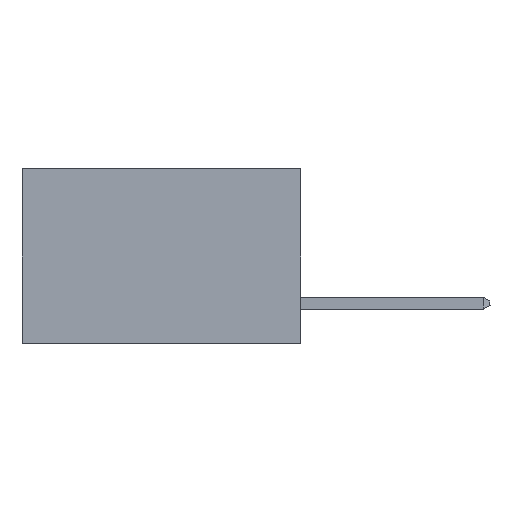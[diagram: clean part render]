
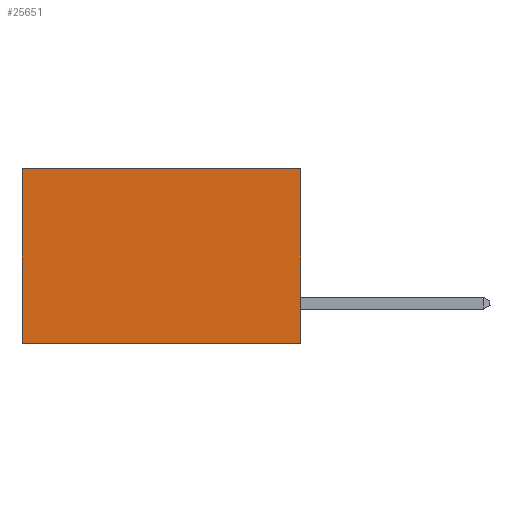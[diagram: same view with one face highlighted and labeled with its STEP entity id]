
A CAD part, left-side view. The second image highlights one B-rep face of the part: STEP entity #25651.
In plain terms, the highlighted planar face has unit normal (-1, 0, 0).
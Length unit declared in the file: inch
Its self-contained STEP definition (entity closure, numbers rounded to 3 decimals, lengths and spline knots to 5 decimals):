
#2387 = DIRECTION ( 'NONE',  ( 0., 0., -1. ) ) ;
#3054 = LINE ( 'NONE', #18910, #8202 ) ;
#3351 = EDGE_CURVE ( 'NONE', #3638, #4696, #25672, .T. ) ;
#3638 = VERTEX_POINT ( 'NONE', #5521 ) ;
#4696 = VERTEX_POINT ( 'NONE', #24232 ) ;
#5521 = CARTESIAN_POINT ( 'NONE',  ( 0.277, 0.59, 0. ) ) ;
#5921 = EDGE_CURVE ( 'NONE', #14532, #13991, #19021, .T. ) ;
#8202 = VECTOR ( 'NONE', #10295, 39.37008 ) ;
#9081 = DIRECTION ( 'NONE',  ( 0., 1., 0. ) ) ;
#9357 = CARTESIAN_POINT ( 'NONE',  ( 0.277, 0., -0.37 ) ) ;
#9392 = DIRECTION ( 'NONE',  ( 0., 0., -1. ) ) ;
#10214 = CARTESIAN_POINT ( 'NONE',  ( 0.277, 0., -0.37 ) ) ;
#10295 = DIRECTION ( 'NONE',  ( 0., 1., 0. ) ) ;
#11692 = ORIENTED_EDGE ( 'NONE', *, *, #3351, .T. ) ;
#12335 = DIRECTION ( 'NONE',  ( 0., 0., -1. ) ) ;
#12855 = EDGE_CURVE ( 'NONE', #13991, #4696, #24137, .T. ) ;
#13382 = VECTOR ( 'NONE', #2387, 39.37008 ) ;
#13991 = VERTEX_POINT ( 'NONE', #21744 ) ;
#14090 = ORIENTED_EDGE ( 'NONE', *, *, #12855, .F. ) ;
#14532 = VERTEX_POINT ( 'NONE', #27782 ) ;
#15339 = FACE_OUTER_BOUND ( 'NONE', #27170, .T. ) ;
#15500 = CARTESIAN_POINT ( 'NONE',  ( 0.277, 0., -0.37 ) ) ;
#16653 = PLANE ( 'NONE',  #22924 ) ;
#18342 = VECTOR ( 'NONE', #9392, 39.37008 ) ;
#18575 = EDGE_CURVE ( 'NONE', #14532, #3638, #3054, .T. ) ;
#18910 = CARTESIAN_POINT ( 'NONE',  ( 0.277, 0., 0. ) ) ;
#19021 = LINE ( 'NONE', #9357, #18342 ) ;
#19852 = ORIENTED_EDGE ( 'NONE', *, *, #5921, .F. ) ;
#21059 = ORIENTED_EDGE ( 'NONE', *, *, #18575, .T. ) ;
#21744 = CARTESIAN_POINT ( 'NONE',  ( 0.277, 0., -0.37 ) ) ;
#22924 = AXIS2_PLACEMENT_3D ( 'NONE', #10214, #25407, #12335 ) ;
#23452 = VECTOR ( 'NONE', #9081, 39.37008 ) ;
#24137 = LINE ( 'NONE', #15500, #23452 ) ;
#24232 = CARTESIAN_POINT ( 'NONE',  ( 0.277, 0.59, -0.37 ) ) ;
#25407 = DIRECTION ( 'NONE',  ( 1., 0., 0. ) ) ;
#25651 = ADVANCED_FACE ( 'NONE', ( #15339 ), #16653, .F. ) ;
#25672 = LINE ( 'NONE', #26267, #13382 ) ;
#26267 = CARTESIAN_POINT ( 'NONE',  ( 0.277, 0.59, -0.37 ) ) ;
#27170 = EDGE_LOOP ( 'NONE', ( #11692, #14090, #19852, #21059 ) ) ;
#27782 = CARTESIAN_POINT ( 'NONE',  ( 0.277, 0., 0. ) ) ;
